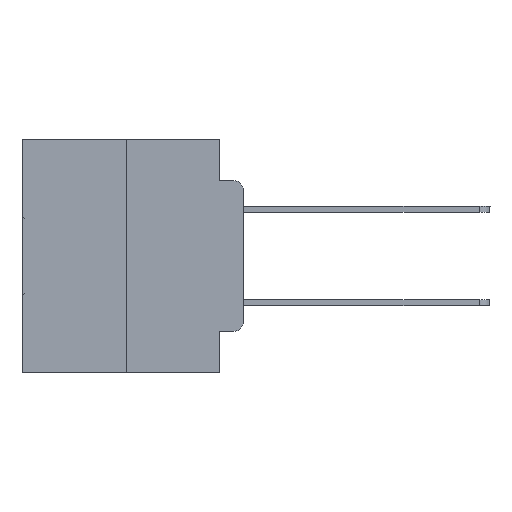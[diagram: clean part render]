
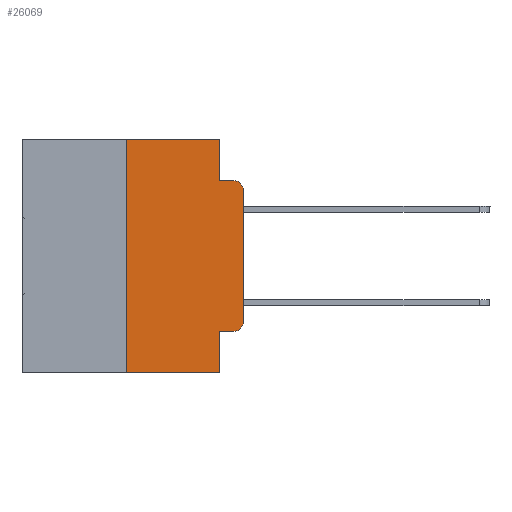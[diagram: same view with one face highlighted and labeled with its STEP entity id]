
A CAD part, left-side view. The second image highlights one B-rep face of the part: STEP entity #26069.
In plain terms, the highlighted planar face has unit normal (-1, 0, 0).
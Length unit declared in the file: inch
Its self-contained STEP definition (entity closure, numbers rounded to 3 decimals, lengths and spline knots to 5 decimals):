
#320 = VECTOR ( 'NONE', #25884, 39.37008 ) ;
#863 = VERTEX_POINT ( 'NONE', #30273 ) ;
#1496 = CARTESIAN_POINT ( 'NONE',  ( 0., 0.473, -0.5 ) ) ;
#1634 = ORIENTED_EDGE ( 'NONE', *, *, #25132, .F. ) ;
#2052 = ORIENTED_EDGE ( 'NONE', *, *, #20353, .T. ) ;
#2785 = VECTOR ( 'NONE', #10252, 39.37008 ) ;
#4082 = ORIENTED_EDGE ( 'NONE', *, *, #29462, .T. ) ;
#4116 = DIRECTION ( 'NONE',  ( 0., -1., 0. ) ) ;
#5150 = LINE ( 'NONE', #19075, #11037 ) ;
#5456 = CARTESIAN_POINT ( 'NONE',  ( 0., 0.25, 0. ) ) ;
#6813 = DIRECTION ( 'NONE',  ( 0., 0., -1. ) ) ;
#7278 = LINE ( 'NONE', #1496, #30159 ) ;
#7341 = EDGE_CURVE ( 'NONE', #10308, #16366, #7679, .T. ) ;
#7679 = LINE ( 'NONE', #28102, #19941 ) ;
#8416 = DIRECTION ( 'NONE',  ( -1., 0., 0. ) ) ;
#8573 = VECTOR ( 'NONE', #16666, 39.37008 ) ;
#8713 = VERTEX_POINT ( 'NONE', #16093 ) ;
#9246 = ORIENTED_EDGE ( 'NONE', *, *, #13176, .F. ) ;
#9992 = VECTOR ( 'NONE', #10980, 39.37008 ) ;
#10106 = EDGE_CURVE ( 'NONE', #15587, #15717, #15018, .T. ) ;
#10252 = DIRECTION ( 'NONE',  ( 0., 0., 1. ) ) ;
#10308 = VERTEX_POINT ( 'NONE', #26165 ) ;
#10887 = CARTESIAN_POINT ( 'NONE',  ( 0., 0., -0.3915 ) ) ;
#10980 = DIRECTION ( 'NONE',  ( 0., 0., 1. ) ) ;
#11037 = VECTOR ( 'NONE', #6813, 39.37008 ) ;
#11289 = EDGE_CURVE ( 'NONE', #27976, #27919, #22502, .T. ) ;
#12307 = ORIENTED_EDGE ( 'NONE', *, *, #25909, .F. ) ;
#13176 = EDGE_CURVE ( 'NONE', #27919, #10308, #18606, .T. ) ;
#13805 = LINE ( 'NONE', #25983, #320 ) ;
#14315 = CARTESIAN_POINT ( 'NONE',  ( 0., 0.02, -0.3915 ) ) ;
#14830 = DIRECTION ( 'NONE',  ( 1., 0., 0. ) ) ;
#15018 = LINE ( 'NONE', #30400, #9992 ) ;
#15123 = LINE ( 'NONE', #28604, #8573 ) ;
#15269 = AXIS2_PLACEMENT_3D ( 'NONE', #23010, #8416, #25458 ) ;
#15587 = VERTEX_POINT ( 'NONE', #10887 ) ;
#15681 = CARTESIAN_POINT ( 'NONE',  ( 0., 0.25, -0.5 ) ) ;
#15717 = VERTEX_POINT ( 'NONE', #28397 ) ;
#15801 = EDGE_CURVE ( 'NONE', #20087, #8713, #15123, .T. ) ;
#15807 = ORIENTED_EDGE ( 'NONE', *, *, #11289, .F. ) ;
#16088 = DIRECTION ( 'NONE',  ( 0., -1., 0. ) ) ;
#16093 = CARTESIAN_POINT ( 'NONE',  ( 0., 0.02, -0.4115 ) ) ;
#16366 = VERTEX_POINT ( 'NONE', #29221 ) ;
#16666 = DIRECTION ( 'NONE',  ( 0., -1., 0. ) ) ;
#16754 = DIRECTION ( 'NONE',  ( 0., 0., -1. ) ) ;
#16923 = AXIS2_PLACEMENT_3D ( 'NONE', #14315, #31213, #16754 ) ;
#17302 = CIRCLE ( 'NONE', #15269, 0.02 ) ;
#17766 = EDGE_CURVE ( 'NONE', #15717, #863, #17302, .T. ) ;
#18199 = ORIENTED_EDGE ( 'NONE', *, *, #10106, .T. ) ;
#18606 = LINE ( 'NONE', #30549, #24254 ) ;
#19075 = CARTESIAN_POINT ( 'NONE',  ( 0., 0.051, 0. ) ) ;
#19536 = VERTEX_POINT ( 'NONE', #20818 ) ;
#19688 = CARTESIAN_POINT ( 'NONE',  ( 0., 0.473, 0. ) ) ;
#19941 = VECTOR ( 'NONE', #30520, 39.37008 ) ;
#20087 = VERTEX_POINT ( 'NONE', #22893 ) ;
#20196 = FACE_OUTER_BOUND ( 'NONE', #27352, .T. ) ;
#20353 = EDGE_CURVE ( 'NONE', #8713, #15587, #22792, .T. ) ;
#20818 = CARTESIAN_POINT ( 'NONE',  ( 0., 0.051, -0.5 ) ) ;
#21464 = ORIENTED_EDGE ( 'NONE', *, *, #7341, .F. ) ;
#22139 = PLANE ( 'NONE',  #24080 ) ;
#22502 = LINE ( 'NONE', #23209, #2785 ) ;
#22792 = CIRCLE ( 'NONE', #16923, 0.02 ) ;
#22893 = CARTESIAN_POINT ( 'NONE',  ( 0., 0.051, -0.4115 ) ) ;
#23010 = CARTESIAN_POINT ( 'NONE',  ( 0., 0.02, -0.1085 ) ) ;
#23209 = CARTESIAN_POINT ( 'NONE',  ( 0., 0.25, 0. ) ) ;
#24080 = AXIS2_PLACEMENT_3D ( 'NONE', #19688, #14830, #24537 ) ;
#24254 = VECTOR ( 'NONE', #16088, 39.37008 ) ;
#24537 = DIRECTION ( 'NONE',  ( 0., 0., -1. ) ) ;
#25132 = EDGE_CURVE ( 'NONE', #16366, #863, #13805, .T. ) ;
#25458 = DIRECTION ( 'NONE',  ( 0., 0., -1. ) ) ;
#25884 = DIRECTION ( 'NONE',  ( 0., -1., 0. ) ) ;
#25909 = EDGE_CURVE ( 'NONE', #20087, #19536, #5150, .T. ) ;
#25983 = CARTESIAN_POINT ( 'NONE',  ( 0., 0.051, -0.0885 ) ) ;
#26069 = ADVANCED_FACE ( 'NONE', ( #20196 ), #22139, .F. ) ;
#26165 = CARTESIAN_POINT ( 'NONE',  ( 0., 0.051, 0. ) ) ;
#27112 = ORIENTED_EDGE ( 'NONE', *, *, #17766, .T. ) ;
#27352 = EDGE_LOOP ( 'NONE', ( #18199, #27112, #1634, #21464, #9246, #15807, #4082, #12307, #31641, #2052 ) ) ;
#27919 = VERTEX_POINT ( 'NONE', #5456 ) ;
#27976 = VERTEX_POINT ( 'NONE', #15681 ) ;
#28102 = CARTESIAN_POINT ( 'NONE',  ( 0., 0.051, 0. ) ) ;
#28397 = CARTESIAN_POINT ( 'NONE',  ( 0., 0., -0.1085 ) ) ;
#28604 = CARTESIAN_POINT ( 'NONE',  ( 0., 0.051, -0.4115 ) ) ;
#29221 = CARTESIAN_POINT ( 'NONE',  ( 0., 0.051, -0.0885 ) ) ;
#29462 = EDGE_CURVE ( 'NONE', #27976, #19536, #7278, .T. ) ;
#30159 = VECTOR ( 'NONE', #4116, 39.37008 ) ;
#30273 = CARTESIAN_POINT ( 'NONE',  ( 0., 0.02, -0.0885 ) ) ;
#30400 = CARTESIAN_POINT ( 'NONE',  ( 0., 0., 0. ) ) ;
#30520 = DIRECTION ( 'NONE',  ( 0., 0., -1. ) ) ;
#30549 = CARTESIAN_POINT ( 'NONE',  ( 0., 0.473, 0. ) ) ;
#31213 = DIRECTION ( 'NONE',  ( -1., 0., 0. ) ) ;
#31641 = ORIENTED_EDGE ( 'NONE', *, *, #15801, .T. ) ;
